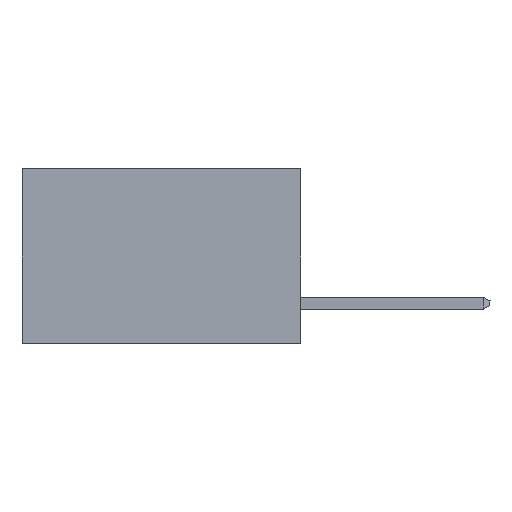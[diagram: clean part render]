
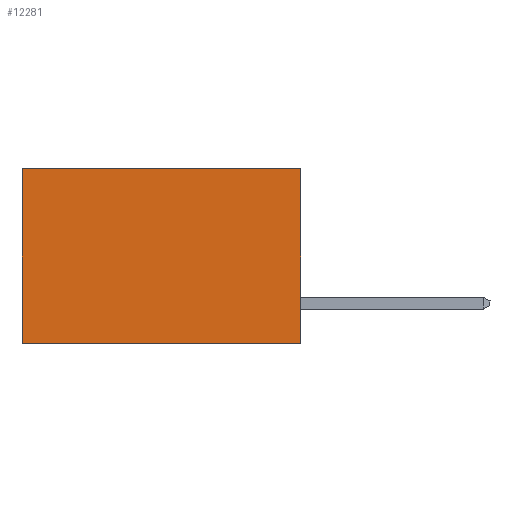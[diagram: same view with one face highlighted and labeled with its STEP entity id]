
A CAD part, left-side view. The second image highlights one B-rep face of the part: STEP entity #12281.
In plain terms, the highlighted planar face has unit normal (-1, 0, 0).
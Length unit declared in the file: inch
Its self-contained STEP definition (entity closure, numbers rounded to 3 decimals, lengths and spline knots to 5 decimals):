
#230 = DIRECTION ( 'NONE',  ( 0., 1., 0. ) ) ;
#425 = CARTESIAN_POINT ( 'NONE',  ( 0.277, 0., -0.37 ) ) ;
#867 = CARTESIAN_POINT ( 'NONE',  ( 0.277, 0., -0.37 ) ) ;
#912 = DIRECTION ( 'NONE',  ( 1., 0., 0. ) ) ;
#2103 = VERTEX_POINT ( 'NONE', #9591 ) ;
#2173 = LINE ( 'NONE', #8712, #4075 ) ;
#2383 = LINE ( 'NONE', #10428, #4858 ) ;
#2574 = EDGE_CURVE ( 'NONE', #7931, #7857, #7253, .T. ) ;
#3212 = VERTEX_POINT ( 'NONE', #8078 ) ;
#4075 = VECTOR ( 'NONE', #7516, 39.37008 ) ;
#4094 = CARTESIAN_POINT ( 'NONE',  ( 0.277, 0., -0.37 ) ) ;
#4202 = EDGE_CURVE ( 'NONE', #3212, #7931, #2383, .T. ) ;
#4463 = CARTESIAN_POINT ( 'NONE',  ( 0.277, 0.59, -0.37 ) ) ;
#4656 = VECTOR ( 'NONE', #230, 39.37008 ) ;
#4858 = VECTOR ( 'NONE', #6382, 39.37008 ) ;
#4982 = ORIENTED_EDGE ( 'NONE', *, *, #11081, .T. ) ;
#4996 = ORIENTED_EDGE ( 'NONE', *, *, #2574, .F. ) ;
#5069 = ORIENTED_EDGE ( 'NONE', *, *, #4202, .F. ) ;
#5071 = ORIENTED_EDGE ( 'NONE', *, *, #5745, .T. ) ;
#5666 = EDGE_LOOP ( 'NONE', ( #4982, #4996, #5069, #5071 ) ) ;
#5745 = EDGE_CURVE ( 'NONE', #3212, #2103, #2173, .T. ) ;
#6382 = DIRECTION ( 'NONE',  ( 0., 0., -1. ) ) ;
#6695 = DIRECTION ( 'NONE',  ( 0., 0., -1. ) ) ;
#6699 = PLANE ( 'NONE',  #11511 ) ;
#6855 = LINE ( 'NONE', #12555, #9456 ) ;
#7253 = LINE ( 'NONE', #425, #4656 ) ;
#7516 = DIRECTION ( 'NONE',  ( 0., 1., 0. ) ) ;
#7658 = DIRECTION ( 'NONE',  ( 0., 0., -1. ) ) ;
#7857 = VERTEX_POINT ( 'NONE', #4463 ) ;
#7931 = VERTEX_POINT ( 'NONE', #4094 ) ;
#8078 = CARTESIAN_POINT ( 'NONE',  ( 0.277, 0., 0. ) ) ;
#8174 = FACE_OUTER_BOUND ( 'NONE', #5666, .T. ) ;
#8712 = CARTESIAN_POINT ( 'NONE',  ( 0.277, 0., 0. ) ) ;
#9456 = VECTOR ( 'NONE', #6695, 39.37008 ) ;
#9591 = CARTESIAN_POINT ( 'NONE',  ( 0.277, 0.59, 0. ) ) ;
#10428 = CARTESIAN_POINT ( 'NONE',  ( 0.277, 0., -0.37 ) ) ;
#11081 = EDGE_CURVE ( 'NONE', #2103, #7857, #6855, .T. ) ;
#11511 = AXIS2_PLACEMENT_3D ( 'NONE', #867, #912, #7658 ) ;
#12281 = ADVANCED_FACE ( 'NONE', ( #8174 ), #6699, .F. ) ;
#12555 = CARTESIAN_POINT ( 'NONE',  ( 0.277, 0.59, -0.37 ) ) ;
